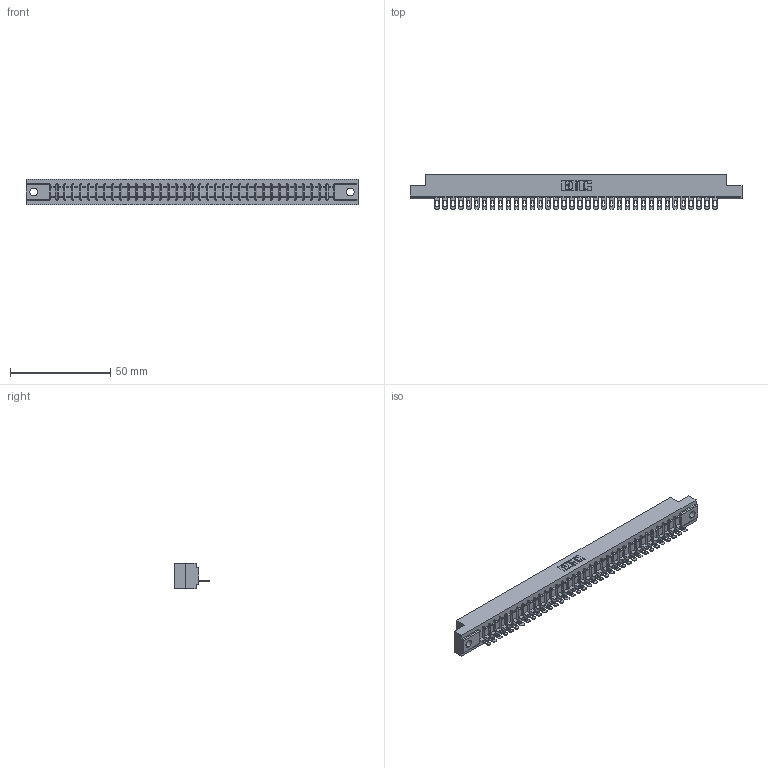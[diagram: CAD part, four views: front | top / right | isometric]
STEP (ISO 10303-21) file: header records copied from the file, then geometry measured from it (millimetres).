
FILE_DESCRIPTION (( 'STEP AP203' ), '1' );
FILE_NAME ('357-036-401-104.STEP', '2020-10-02T17:11:14', ( '' ), ( '' ), 'SwSTEP 2.0', 'SolidWorks 2020', '' );
FILE_SCHEMA (( 'CONFIG_CONTROL_DESIGN' ));
Length unit declared in the file: inch
Products named in the file (3): 307-290-002_501; 357-036-401-104; 307 Part_.156 Dia Mounting Holes
Assembly tree (37 placements, depth 2):
  357-036-401-104
    307 Part_.156 Dia Mounting Holes
    307-290-002_501  x36
Bounding box: 165.66 x 17.42 x 12.7 mm (x, y, z)
Volume: 17608.3 mm3; surface area: 22087.5 mm2
Topology: 37 solids, 37 shells, 2905 faces, 8927 edges, 5850 vertices
Faces by surface type: plane 1668, cylinder 1163, sphere 74
Entity records: 32814 total; most frequent: CARTESIAN_POINT 5538, ORIENTED_EDGE 5526, DIRECTION 5379, EDGE_CURVE 2763, LINE 2117, VECTOR 2117, VERTEX_POINT 1790, AXIS2_PLACEMENT_3D 1631
